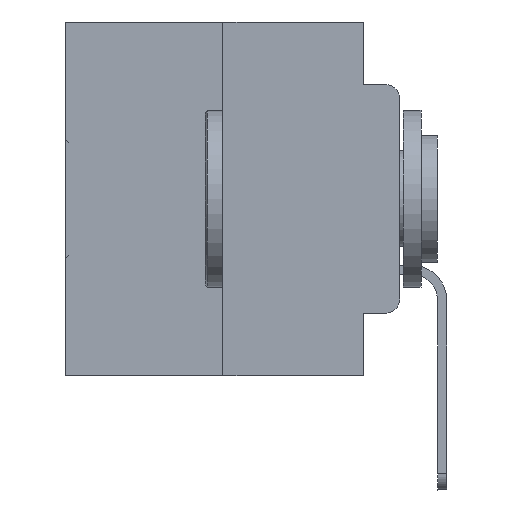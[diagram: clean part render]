
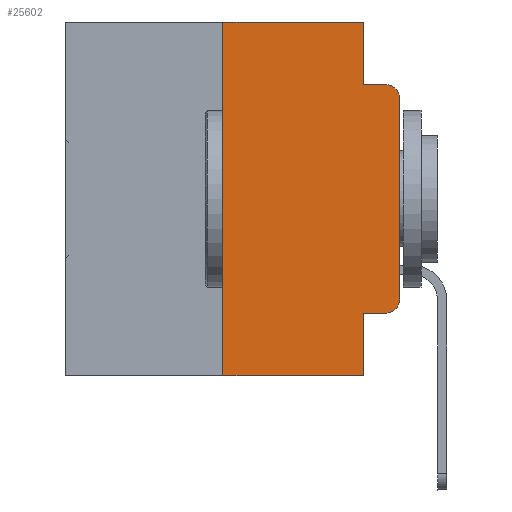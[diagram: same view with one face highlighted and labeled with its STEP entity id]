
A CAD part, left-side view. The second image highlights one B-rep face of the part: STEP entity #25602.
In plain terms, the highlighted planar face has unit normal (-1, 0, 0).
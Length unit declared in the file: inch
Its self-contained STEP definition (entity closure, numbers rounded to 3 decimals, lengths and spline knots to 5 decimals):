
#149 = CARTESIAN_POINT ( 'NONE',  ( 0., 0.051, -0.4115 ) ) ;
#1090 = DIRECTION ( 'NONE',  ( 0., 0., 1. ) ) ;
#1315 = DIRECTION ( 'NONE',  ( 0., 0., -1. ) ) ;
#1382 = LINE ( 'NONE', #1702, #22038 ) ;
#1464 = EDGE_CURVE ( 'NONE', #27069, #6917, #31085, .T. ) ;
#1644 = LINE ( 'NONE', #30607, #3142 ) ;
#1702 = CARTESIAN_POINT ( 'NONE',  ( 0., 0.051, -0.4115 ) ) ;
#2059 = LINE ( 'NONE', #17084, #12002 ) ;
#2201 = ORIENTED_EDGE ( 'NONE', *, *, #3294, .T. ) ;
#2544 = CARTESIAN_POINT ( 'NONE',  ( 0., 0.051, -0.5 ) ) ;
#2824 = EDGE_CURVE ( 'NONE', #7148, #12845, #25444, .T. ) ;
#2913 = FACE_OUTER_BOUND ( 'NONE', #15230, .T. ) ;
#3018 = VECTOR ( 'NONE', #29330, 39.37008 ) ;
#3142 = VECTOR ( 'NONE', #15895, 39.37008 ) ;
#3294 = EDGE_CURVE ( 'NONE', #26420, #6916, #1382, .T. ) ;
#4102 = EDGE_CURVE ( 'NONE', #6916, #27069, #13810, .T. ) ;
#4808 = ORIENTED_EDGE ( 'NONE', *, *, #16603, .T. ) ;
#5467 = DIRECTION ( 'NONE',  ( 0., 0., -1. ) ) ;
#5490 = ORIENTED_EDGE ( 'NONE', *, *, #11300, .F. ) ;
#5523 = CARTESIAN_POINT ( 'NONE',  ( 0., 0.25, -0.5 ) ) ;
#5987 = ORIENTED_EDGE ( 'NONE', *, *, #18998, .F. ) ;
#6315 = DIRECTION ( 'NONE',  ( 0., -1., 0. ) ) ;
#6894 = VECTOR ( 'NONE', #6315, 39.37008 ) ;
#6916 = VERTEX_POINT ( 'NONE', #12177 ) ;
#6917 = VERTEX_POINT ( 'NONE', #28501 ) ;
#7148 = VERTEX_POINT ( 'NONE', #29841 ) ;
#7243 = AXIS2_PLACEMENT_3D ( 'NONE', #15988, #30237, #11259 ) ;
#7779 = VERTEX_POINT ( 'NONE', #2544 ) ;
#7923 = CARTESIAN_POINT ( 'NONE',  ( 0., 0.051, 0. ) ) ;
#8317 = CARTESIAN_POINT ( 'NONE',  ( 0., 0.051, 0. ) ) ;
#8697 = DIRECTION ( 'NONE',  ( 0., -1., 0. ) ) ;
#8803 = ORIENTED_EDGE ( 'NONE', *, *, #2824, .F. ) ;
#9867 = EDGE_CURVE ( 'NONE', #26420, #7779, #13357, .T. ) ;
#11259 = DIRECTION ( 'NONE',  ( 0., 0., -1. ) ) ;
#11300 = EDGE_CURVE ( 'NONE', #21433, #13266, #20089, .T. ) ;
#11625 = DIRECTION ( 'NONE',  ( 0., 0., 1. ) ) ;
#11765 = EDGE_CURVE ( 'NONE', #12511, #7148, #1644, .T. ) ;
#12002 = VECTOR ( 'NONE', #12352, 39.37008 ) ;
#12177 = CARTESIAN_POINT ( 'NONE',  ( 0., 0.02, -0.4115 ) ) ;
#12352 = DIRECTION ( 'NONE',  ( 0., -1., 0. ) ) ;
#12428 = DIRECTION ( 'NONE',  ( 1., 0., 0. ) ) ;
#12511 = VERTEX_POINT ( 'NONE', #7923 ) ;
#12747 = CARTESIAN_POINT ( 'NONE',  ( 0., 0.473, 0. ) ) ;
#12845 = VERTEX_POINT ( 'NONE', #24018 ) ;
#12903 = ORIENTED_EDGE ( 'NONE', *, *, #11765, .F. ) ;
#13266 = VERTEX_POINT ( 'NONE', #22093 ) ;
#13357 = LINE ( 'NONE', #8317, #21619 ) ;
#13810 = CIRCLE ( 'NONE', #7243, 0.02 ) ;
#14963 = PLANE ( 'NONE',  #24271 ) ;
#15230 = EDGE_LOOP ( 'NONE', ( #17232, #18458, #8803, #12903, #5987, #5490, #4808, #21611, #2201, #28747 ) ) ;
#15895 = DIRECTION ( 'NONE',  ( 0., 0., -1. ) ) ;
#15963 = EDGE_CURVE ( 'NONE', #6917, #12845, #24104, .T. ) ;
#15988 = CARTESIAN_POINT ( 'NONE',  ( 0., 0.02, -0.3915 ) ) ;
#16603 = EDGE_CURVE ( 'NONE', #21433, #7779, #2059, .T. ) ;
#16865 = DIRECTION ( 'NONE',  ( 0., 0., -1. ) ) ;
#16988 = CARTESIAN_POINT ( 'NONE',  ( 0., 0.473, 0. ) ) ;
#17084 = CARTESIAN_POINT ( 'NONE',  ( 0., 0.473, -0.5 ) ) ;
#17232 = ORIENTED_EDGE ( 'NONE', *, *, #1464, .T. ) ;
#18458 = ORIENTED_EDGE ( 'NONE', *, *, #15963, .T. ) ;
#18998 = EDGE_CURVE ( 'NONE', #13266, #12511, #31228, .T. ) ;
#20089 = LINE ( 'NONE', #20411, #26248 ) ;
#20411 = CARTESIAN_POINT ( 'NONE',  ( 0., 0.25, 0. ) ) ;
#20632 = CARTESIAN_POINT ( 'NONE',  ( 0., 0.02, -0.1085 ) ) ;
#21433 = VERTEX_POINT ( 'NONE', #5523 ) ;
#21611 = ORIENTED_EDGE ( 'NONE', *, *, #9867, .F. ) ;
#21619 = VECTOR ( 'NONE', #1315, 39.37008 ) ;
#22038 = VECTOR ( 'NONE', #8697, 39.37008 ) ;
#22093 = CARTESIAN_POINT ( 'NONE',  ( 0., 0.25, 0. ) ) ;
#22593 = AXIS2_PLACEMENT_3D ( 'NONE', #20632, #27136, #5467 ) ;
#22918 = CARTESIAN_POINT ( 'NONE',  ( 0., 0.051, -0.0885 ) ) ;
#23162 = CARTESIAN_POINT ( 'NONE',  ( 0., 0., -0.3915 ) ) ;
#24018 = CARTESIAN_POINT ( 'NONE',  ( 0., 0.02, -0.0885 ) ) ;
#24104 = CIRCLE ( 'NONE', #22593, 0.02 ) ;
#24271 = AXIS2_PLACEMENT_3D ( 'NONE', #12747, #12428, #16865 ) ;
#25444 = LINE ( 'NONE', #22918, #6894 ) ;
#25602 = ADVANCED_FACE ( 'NONE', ( #2913 ), #14963, .F. ) ;
#26248 = VECTOR ( 'NONE', #1090, 39.37008 ) ;
#26420 = VERTEX_POINT ( 'NONE', #149 ) ;
#27069 = VERTEX_POINT ( 'NONE', #23162 ) ;
#27136 = DIRECTION ( 'NONE',  ( -1., 0., 0. ) ) ;
#27139 = VECTOR ( 'NONE', #11625, 39.37008 ) ;
#28501 = CARTESIAN_POINT ( 'NONE',  ( 0., 0., -0.1085 ) ) ;
#28747 = ORIENTED_EDGE ( 'NONE', *, *, #4102, .T. ) ;
#29330 = DIRECTION ( 'NONE',  ( 0., -1., 0. ) ) ;
#29841 = CARTESIAN_POINT ( 'NONE',  ( 0., 0.051, -0.0885 ) ) ;
#30237 = DIRECTION ( 'NONE',  ( -1., 0., 0. ) ) ;
#30463 = CARTESIAN_POINT ( 'NONE',  ( 0., 0., 0. ) ) ;
#30607 = CARTESIAN_POINT ( 'NONE',  ( 0., 0.051, 0. ) ) ;
#31085 = LINE ( 'NONE', #30463, #27139 ) ;
#31228 = LINE ( 'NONE', #16988, #3018 ) ;
